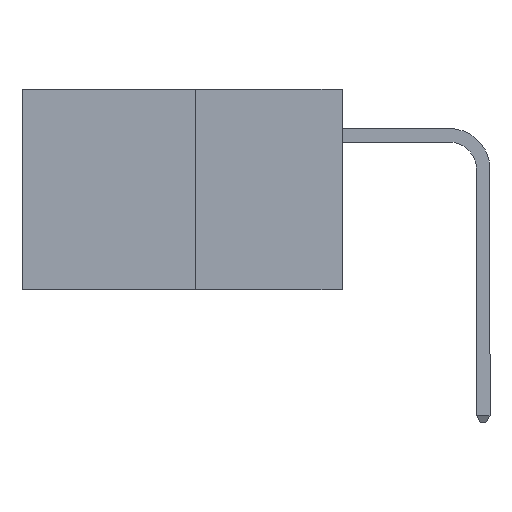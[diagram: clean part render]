
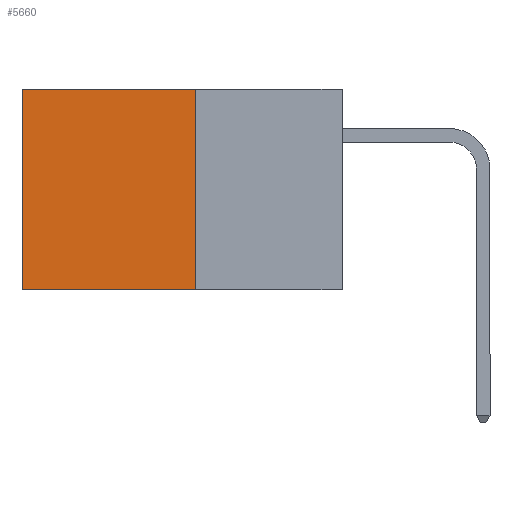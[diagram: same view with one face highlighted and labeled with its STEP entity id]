
A CAD part, left-side view. The second image highlights one B-rep face of the part: STEP entity #5660.
In plain terms, the highlighted planar face has unit normal (-1, 0, 0).
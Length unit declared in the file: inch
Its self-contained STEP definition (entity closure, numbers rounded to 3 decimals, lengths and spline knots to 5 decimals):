
#1268 = ORIENTED_EDGE ( 'NONE', *, *, #19147, .F. ) ;
#1569 = VERTEX_POINT ( 'NONE', #3915 ) ;
#3404 = DIRECTION ( 'NONE',  ( 0., 0., -1. ) ) ;
#3915 = CARTESIAN_POINT ( 'NONE',  ( 0.277, 0.27, -0.37 ) ) ;
#5660 = ADVANCED_FACE ( 'NONE', ( #19951 ), #33229, .F. ) ;
#5874 = LINE ( 'NONE', #10735, #20006 ) ;
#7115 = EDGE_LOOP ( 'NONE', ( #27016, #20469, #1268, #25639 ) ) ;
#7807 = AXIS2_PLACEMENT_3D ( 'NONE', #12164, #30677, #14820 ) ;
#8522 = VECTOR ( 'NONE', #19645, 39.37008 ) ;
#8984 = CARTESIAN_POINT ( 'NONE',  ( 0.277, 0.59, -0.37 ) ) ;
#9014 = CARTESIAN_POINT ( 'NONE',  ( 0.277, 0.59, 0. ) ) ;
#9385 = LINE ( 'NONE', #8984, #8522 ) ;
#9451 = VECTOR ( 'NONE', #30070, 39.37008 ) ;
#9717 = VECTOR ( 'NONE', #3404, 39.37008 ) ;
#10267 = LINE ( 'NONE', #16835, #9451 ) ;
#10735 = CARTESIAN_POINT ( 'NONE',  ( 0.277, 0.27, -0.37 ) ) ;
#12164 = CARTESIAN_POINT ( 'NONE',  ( 0.277, 0.27, -0.37 ) ) ;
#13793 = VERTEX_POINT ( 'NONE', #32049 ) ;
#14820 = DIRECTION ( 'NONE',  ( 0., 0., -1. ) ) ;
#15777 = VERTEX_POINT ( 'NONE', #19163 ) ;
#15827 = EDGE_CURVE ( 'NONE', #13793, #17995, #10267, .T. ) ;
#16669 = EDGE_CURVE ( 'NONE', #17995, #15777, #9385, .T. ) ;
#16835 = CARTESIAN_POINT ( 'NONE',  ( 0.277, 0.27, 0. ) ) ;
#17995 = VERTEX_POINT ( 'NONE', #9014 ) ;
#18598 = DIRECTION ( 'NONE',  ( 0., 1., 0. ) ) ;
#19147 = EDGE_CURVE ( 'NONE', #13793, #1569, #23763, .T. ) ;
#19163 = CARTESIAN_POINT ( 'NONE',  ( 0.277, 0.59, -0.37 ) ) ;
#19645 = DIRECTION ( 'NONE',  ( 0., 0., -1. ) ) ;
#19869 = EDGE_CURVE ( 'NONE', #1569, #15777, #5874, .T. ) ;
#19951 = FACE_OUTER_BOUND ( 'NONE', #7115, .T. ) ;
#20006 = VECTOR ( 'NONE', #18598, 39.37008 ) ;
#20469 = ORIENTED_EDGE ( 'NONE', *, *, #19869, .F. ) ;
#22013 = CARTESIAN_POINT ( 'NONE',  ( 0.277, 0.27, -0.37 ) ) ;
#23763 = LINE ( 'NONE', #22013, #9717 ) ;
#25639 = ORIENTED_EDGE ( 'NONE', *, *, #15827, .T. ) ;
#27016 = ORIENTED_EDGE ( 'NONE', *, *, #16669, .T. ) ;
#30070 = DIRECTION ( 'NONE',  ( 0., 1., 0. ) ) ;
#30677 = DIRECTION ( 'NONE',  ( 1., 0., 0. ) ) ;
#32049 = CARTESIAN_POINT ( 'NONE',  ( 0.277, 0.27, 0. ) ) ;
#33229 = PLANE ( 'NONE',  #7807 ) ;
